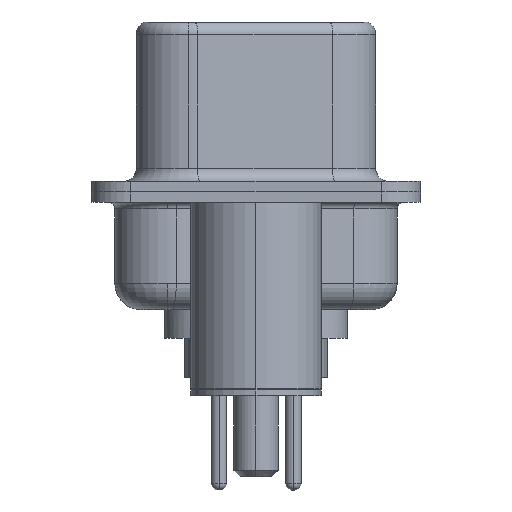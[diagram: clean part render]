
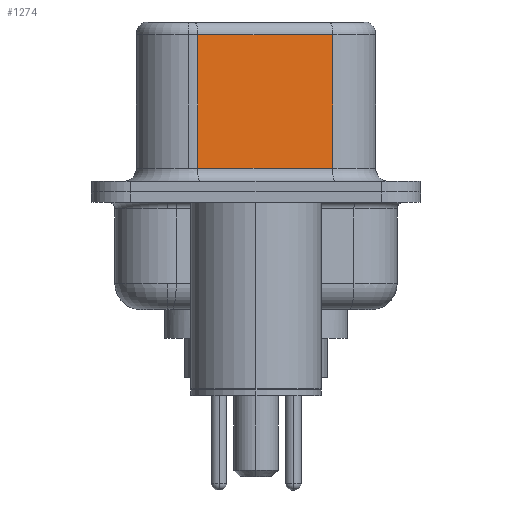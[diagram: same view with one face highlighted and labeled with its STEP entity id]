
A CAD part, left-side view. The second image highlights one B-rep face of the part: STEP entity #1274.
In plain terms, the highlighted planar face has unit normal (-0.985, -0.174, 0).
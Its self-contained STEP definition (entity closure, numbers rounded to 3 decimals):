
#144 = DIRECTION ( 'NONE',  ( -0.174, 0.985, 0. ) ) ;
#1248 = DIRECTION ( 'NONE',  ( 0.174, -0.985, 0. ) ) ;
#1274 = ADVANCED_FACE ( 'NONE', ( #7648 ), #1634, .F. ) ;
#1581 = EDGE_CURVE ( 'NONE', #13568, #18320, #12509, .T. ) ;
#1586 = EDGE_LOOP ( 'NONE', ( #13355, #18592, #3485, #5396 ) ) ;
#1634 = PLANE ( 'NONE',  #9707 ) ;
#2256 = DIRECTION ( 'NONE',  ( 0., 0., -1. ) ) ;
#3348 = VERTEX_POINT ( 'NONE', #10325 ) ;
#3485 = ORIENTED_EDGE ( 'NONE', *, *, #17980, .T. ) ;
#4159 = VECTOR ( 'NONE', #16840, 1000. ) ;
#4235 = EDGE_CURVE ( 'NONE', #18597, #3348, #18236, .T. ) ;
#4387 = CARTESIAN_POINT ( 'NONE',  ( 4.585, -2.927, 6.02 ) ) ;
#4415 = CARTESIAN_POINT ( 'NONE',  ( 3.675, 2.233, 6.52 ) ) ;
#4655 = CARTESIAN_POINT ( 'NONE',  ( 4.585, -2.927, 0.9 ) ) ;
#5396 = ORIENTED_EDGE ( 'NONE', *, *, #1581, .T. ) ;
#7648 = FACE_OUTER_BOUND ( 'NONE', #1586, .T. ) ;
#8375 = CARTESIAN_POINT ( 'NONE',  ( 4.585, -2.927, 0.9 ) ) ;
#9590 = EDGE_CURVE ( 'NONE', #18597, #18320, #12700, .T. ) ;
#9707 = AXIS2_PLACEMENT_3D ( 'NONE', #16923, #19341, #144 ) ;
#9713 = DIRECTION ( 'NONE',  ( -0.174, 0.985, 0. ) ) ;
#10325 = CARTESIAN_POINT ( 'NONE',  ( 3.675, 2.233, 6.02 ) ) ;
#12509 = LINE ( 'NONE', #4655, #18849 ) ;
#12700 = LINE ( 'NONE', #19308, #19534 ) ;
#13355 = ORIENTED_EDGE ( 'NONE', *, *, #9590, .F. ) ;
#13568 = VERTEX_POINT ( 'NONE', #15722 ) ;
#14126 = VECTOR ( 'NONE', #9713, 1000. ) ;
#14572 = CARTESIAN_POINT ( 'NONE',  ( 4.585, -2.927, 6.02 ) ) ;
#15722 = CARTESIAN_POINT ( 'NONE',  ( 3.675, 2.233, 0.9 ) ) ;
#16840 = DIRECTION ( 'NONE',  ( 0., 0., -1. ) ) ;
#16923 = CARTESIAN_POINT ( 'NONE',  ( 4.585, -2.927, 6.52 ) ) ;
#17533 = LINE ( 'NONE', #4415, #4159 ) ;
#17980 = EDGE_CURVE ( 'NONE', #3348, #13568, #17533, .T. ) ;
#18236 = LINE ( 'NONE', #14572, #14126 ) ;
#18320 = VERTEX_POINT ( 'NONE', #8375 ) ;
#18592 = ORIENTED_EDGE ( 'NONE', *, *, #4235, .T. ) ;
#18597 = VERTEX_POINT ( 'NONE', #4387 ) ;
#18849 = VECTOR ( 'NONE', #1248, 1000. ) ;
#19308 = CARTESIAN_POINT ( 'NONE',  ( 4.585, -2.927, 6.52 ) ) ;
#19341 = DIRECTION ( 'NONE',  ( 0.985, 0.174, 0. ) ) ;
#19534 = VECTOR ( 'NONE', #2256, 1000. ) ;
